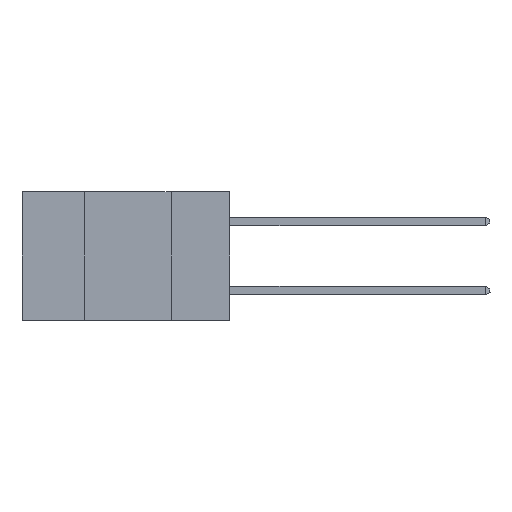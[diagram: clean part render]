
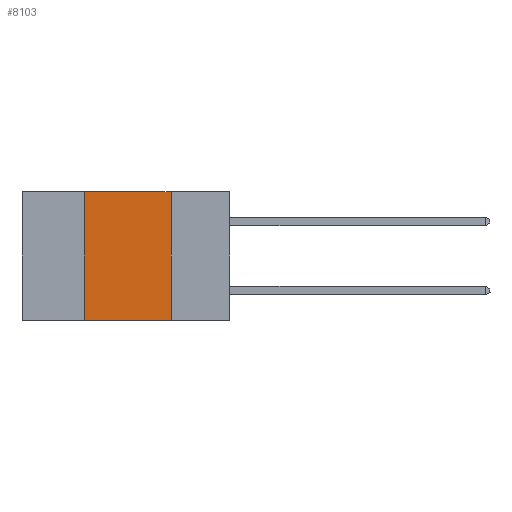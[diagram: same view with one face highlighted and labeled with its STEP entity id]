
A CAD part, left-side view. The second image highlights one B-rep face of the part: STEP entity #8103.
In plain terms, the highlighted planar face has unit normal (-1, 0, 0).
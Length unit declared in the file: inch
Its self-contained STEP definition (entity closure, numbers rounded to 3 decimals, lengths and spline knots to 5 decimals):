
#65 = CARTESIAN_POINT ( 'NONE',  ( 0., 0.42, 0. ) ) ;
#887 = CARTESIAN_POINT ( 'NONE',  ( 0., 0.6, -0.37 ) ) ;
#1605 = ORIENTED_EDGE ( 'NONE', *, *, #7591, .T. ) ;
#2335 = ORIENTED_EDGE ( 'NONE', *, *, #14703, .F. ) ;
#2778 = VECTOR ( 'NONE', #4240, 39.37008 ) ;
#3385 = VECTOR ( 'NONE', #12610, 39.37008 ) ;
#3766 = VERTEX_POINT ( 'NONE', #65 ) ;
#3869 = EDGE_CURVE ( 'NONE', #3766, #7737, #18129, .T. ) ;
#4240 = DIRECTION ( 'NONE',  ( 0., -1., 0. ) ) ;
#4600 = AXIS2_PLACEMENT_3D ( 'NONE', #7978, #17752, #17956 ) ;
#7382 = CARTESIAN_POINT ( 'NONE',  ( 0., 0.6, 0. ) ) ;
#7591 = EDGE_CURVE ( 'NONE', #14865, #18852, #17154, .T. ) ;
#7710 = CARTESIAN_POINT ( 'NONE',  ( 0., 0.17, 0. ) ) ;
#7737 = VERTEX_POINT ( 'NONE', #19298 ) ;
#7978 = CARTESIAN_POINT ( 'NONE',  ( 0., 0.6, 0. ) ) ;
#8103 = ADVANCED_FACE ( 'NONE', ( #16668 ), #8183, .F. ) ;
#8183 = PLANE ( 'NONE',  #4600 ) ;
#11655 = LINE ( 'NONE', #7710, #3385 ) ;
#11724 = VECTOR ( 'NONE', #17201, 39.37008 ) ;
#12174 = CARTESIAN_POINT ( 'NONE',  ( 0., 0.17, -0.37 ) ) ;
#12610 = DIRECTION ( 'NONE',  ( 0., 0., -1. ) ) ;
#12964 = CARTESIAN_POINT ( 'NONE',  ( 0., 0.42, -0.37 ) ) ;
#13561 = DIRECTION ( 'NONE',  ( 0., 0., 1. ) ) ;
#13920 = ORIENTED_EDGE ( 'NONE', *, *, #21435, .F. ) ;
#14703 = EDGE_CURVE ( 'NONE', #7737, #18852, #11655, .T. ) ;
#14865 = VERTEX_POINT ( 'NONE', #12964 ) ;
#14867 = VECTOR ( 'NONE', #13561, 39.37008 ) ;
#15126 = CARTESIAN_POINT ( 'NONE',  ( 0., 0.42, 0. ) ) ;
#15695 = ORIENTED_EDGE ( 'NONE', *, *, #3869, .F. ) ;
#16668 = FACE_OUTER_BOUND ( 'NONE', #21230, .T. ) ;
#16679 = LINE ( 'NONE', #15126, #14867 ) ;
#17154 = LINE ( 'NONE', #887, #2778 ) ;
#17201 = DIRECTION ( 'NONE',  ( 0., -1., 0. ) ) ;
#17752 = DIRECTION ( 'NONE',  ( 1., 0., 0. ) ) ;
#17956 = DIRECTION ( 'NONE',  ( 0., 0., -1. ) ) ;
#18129 = LINE ( 'NONE', #7382, #11724 ) ;
#18852 = VERTEX_POINT ( 'NONE', #12174 ) ;
#19298 = CARTESIAN_POINT ( 'NONE',  ( 0., 0.17, 0. ) ) ;
#21230 = EDGE_LOOP ( 'NONE', ( #2335, #15695, #13920, #1605 ) ) ;
#21435 = EDGE_CURVE ( 'NONE', #14865, #3766, #16679, .T. ) ;
